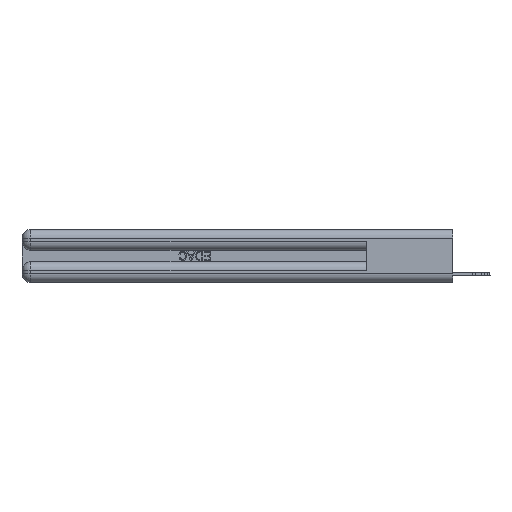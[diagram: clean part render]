
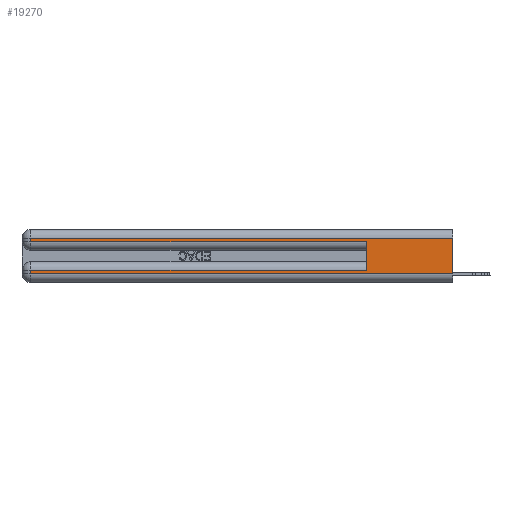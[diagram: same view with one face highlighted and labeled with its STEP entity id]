
A CAD part, left-side view. The second image highlights one B-rep face of the part: STEP entity #19270.
In plain terms, the highlighted planar face has unit normal (-1, 0, 0).
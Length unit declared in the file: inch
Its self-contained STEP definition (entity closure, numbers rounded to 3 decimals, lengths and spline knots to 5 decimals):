
#372 = VECTOR ( 'NONE', #21154, 39.37008 ) ;
#584 = EDGE_CURVE ( 'NONE', #6488, #7298, #21197, .T. ) ;
#1548 = VECTOR ( 'NONE', #34927, 39.37008 ) ;
#2106 = CARTESIAN_POINT ( 'NONE',  ( 0., 0., 0.085 ) ) ;
#2736 = DIRECTION ( 'NONE',  ( 0., 0., -1. ) ) ;
#2767 = LINE ( 'NONE', #3106, #35326 ) ;
#3106 = CARTESIAN_POINT ( 'NONE',  ( 0., 0.6, 0.145 ) ) ;
#3476 = CARTESIAN_POINT ( 'NONE',  ( 0., 0., 0.06 ) ) ;
#4408 = VECTOR ( 'NONE', #5807, 39.37008 ) ;
#5391 = ORIENTED_EDGE ( 'NONE', *, *, #19752, .F. ) ;
#5807 = DIRECTION ( 'NONE',  ( 0., -1., 0. ) ) ;
#5981 = EDGE_CURVE ( 'NONE', #10891, #23189, #7087, .T. ) ;
#6488 = VERTEX_POINT ( 'NONE', #9922 ) ;
#6631 = DIRECTION ( 'NONE',  ( 0., 0., -1. ) ) ;
#6937 = VERTEX_POINT ( 'NONE', #32641 ) ;
#7087 = LINE ( 'NONE', #9782, #1548 ) ;
#7298 = VERTEX_POINT ( 'NONE', #12482 ) ;
#7924 = VECTOR ( 'NONE', #27535, 39.37008 ) ;
#8674 = LINE ( 'NONE', #22503, #4408 ) ;
#9310 = VECTOR ( 'NONE', #29451, 39.37008 ) ;
#9349 = PLANE ( 'NONE',  #34808 ) ;
#9782 = CARTESIAN_POINT ( 'NONE',  ( 0., 2.94, 0.37 ) ) ;
#9922 = CARTESIAN_POINT ( 'NONE',  ( 0., 2.94, 0.285 ) ) ;
#10737 = VECTOR ( 'NONE', #2736, 39.37008 ) ;
#10891 = VERTEX_POINT ( 'NONE', #31696 ) ;
#11139 = VERTEX_POINT ( 'NONE', #3476 ) ;
#12455 = VECTOR ( 'NONE', #6631, 39.37008 ) ;
#12482 = CARTESIAN_POINT ( 'NONE',  ( 0., 0.6, 0.285 ) ) ;
#13460 = CARTESIAN_POINT ( 'NONE',  ( 0., 0.6, 0.085 ) ) ;
#14904 = CARTESIAN_POINT ( 'NONE',  ( 0., 0., 0.31 ) ) ;
#16099 = EDGE_CURVE ( 'NONE', #29170, #7298, #2767, .T. ) ;
#16880 = EDGE_LOOP ( 'NONE', ( #5391, #23508, #26764, #25187, #31426, #25635, #20466, #34709 ) ) ;
#18424 = CARTESIAN_POINT ( 'NONE',  ( 0., 2.94, 0.06 ) ) ;
#18714 = LINE ( 'NONE', #35420, #10737 ) ;
#18724 = EDGE_CURVE ( 'NONE', #29170, #10891, #29586, .T. ) ;
#19270 = ADVANCED_FACE ( 'NONE', ( #33947 ), #9349, .F. ) ;
#19752 = EDGE_CURVE ( 'NONE', #22067, #11139, #18714, .T. ) ;
#20118 = CARTESIAN_POINT ( 'NONE',  ( 0., 2.94, 0.37 ) ) ;
#20313 = DIRECTION ( 'NONE',  ( 1., 0., 0. ) ) ;
#20466 = ORIENTED_EDGE ( 'NONE', *, *, #5981, .T. ) ;
#21154 = DIRECTION ( 'NONE',  ( 0., 1., 0. ) ) ;
#21197 = LINE ( 'NONE', #31957, #9310 ) ;
#22067 = VERTEX_POINT ( 'NONE', #26689 ) ;
#22503 = CARTESIAN_POINT ( 'NONE',  ( 0., 0., 0.06 ) ) ;
#23189 = VERTEX_POINT ( 'NONE', #18424 ) ;
#23357 = CARTESIAN_POINT ( 'NONE',  ( 0., 0., 0.37 ) ) ;
#23508 = ORIENTED_EDGE ( 'NONE', *, *, #24299, .T. ) ;
#24299 = EDGE_CURVE ( 'NONE', #22067, #6937, #31048, .T. ) ;
#24385 = EDGE_CURVE ( 'NONE', #6937, #6488, #31403, .T. ) ;
#25187 = ORIENTED_EDGE ( 'NONE', *, *, #584, .T. ) ;
#25499 = EDGE_CURVE ( 'NONE', #23189, #11139, #8674, .T. ) ;
#25635 = ORIENTED_EDGE ( 'NONE', *, *, #18724, .T. ) ;
#26689 = CARTESIAN_POINT ( 'NONE',  ( 0., 0., 0.31 ) ) ;
#26764 = ORIENTED_EDGE ( 'NONE', *, *, #24385, .T. ) ;
#27535 = DIRECTION ( 'NONE',  ( 0., 1., 0. ) ) ;
#27891 = DIRECTION ( 'NONE',  ( 0., 0., 1. ) ) ;
#29170 = VERTEX_POINT ( 'NONE', #13460 ) ;
#29451 = DIRECTION ( 'NONE',  ( 0., -1., 0. ) ) ;
#29586 = LINE ( 'NONE', #2106, #372 ) ;
#31048 = LINE ( 'NONE', #14904, #7924 ) ;
#31403 = LINE ( 'NONE', #20118, #12455 ) ;
#31426 = ORIENTED_EDGE ( 'NONE', *, *, #16099, .F. ) ;
#31696 = CARTESIAN_POINT ( 'NONE',  ( 0., 2.94, 0.085 ) ) ;
#31957 = CARTESIAN_POINT ( 'NONE',  ( 0., 0., 0.285 ) ) ;
#32641 = CARTESIAN_POINT ( 'NONE',  ( 0., 2.94, 0.31 ) ) ;
#33947 = FACE_OUTER_BOUND ( 'NONE', #16880, .T. ) ;
#34484 = DIRECTION ( 'NONE',  ( 0., 0., -1. ) ) ;
#34709 = ORIENTED_EDGE ( 'NONE', *, *, #25499, .T. ) ;
#34808 = AXIS2_PLACEMENT_3D ( 'NONE', #23357, #20313, #34484 ) ;
#34927 = DIRECTION ( 'NONE',  ( 0., 0., -1. ) ) ;
#35326 = VECTOR ( 'NONE', #27891, 39.37008 ) ;
#35420 = CARTESIAN_POINT ( 'NONE',  ( 0., 0., 0.37 ) ) ;
